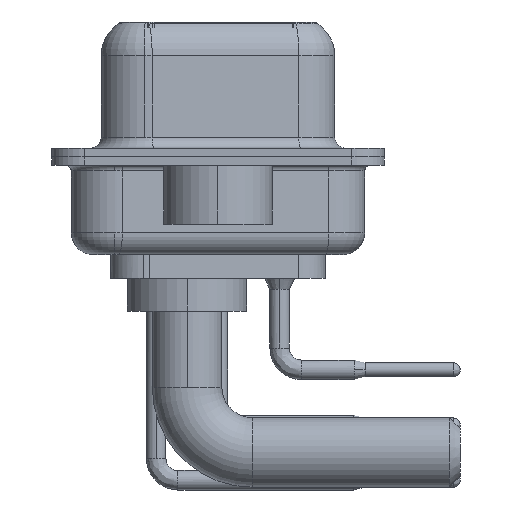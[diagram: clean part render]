
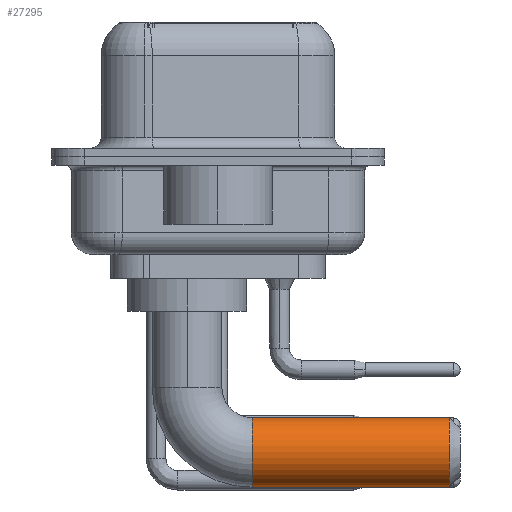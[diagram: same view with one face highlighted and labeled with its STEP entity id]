
A CAD part, left-side view. The second image highlights one B-rep face of the part: STEP entity #27295.
In plain terms, the highlighted cylindrical face has radius 1.6 mm (diameter 3.2 mm), a partial arc.
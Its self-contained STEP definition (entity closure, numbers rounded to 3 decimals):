
#317 = CARTESIAN_POINT ( 'NONE',  ( 0., -12.07, -8.1 ) ) ;
#1496 = DIRECTION ( 'NONE',  ( 0., -1., 0. ) ) ;
#2764 = ORIENTED_EDGE ( 'NONE', *, *, #27923, .F. ) ;
#2910 = DIRECTION ( 'NONE',  ( 0., 1., 0. ) ) ;
#3071 = DIRECTION ( 'NONE',  ( 0., -1., 0. ) ) ;
#3340 = VECTOR ( 'NONE', #7880, 1000. ) ;
#6502 = VERTEX_POINT ( 'NONE', #18603 ) ;
#7880 = DIRECTION ( 'NONE',  ( 0., -1., 0. ) ) ;
#8412 = CARTESIAN_POINT ( 'NONE',  ( 0., -3., -6.5 ) ) ;
#8477 = ORIENTED_EDGE ( 'NONE', *, *, #17776, .T. ) ;
#10902 = CYLINDRICAL_SURFACE ( 'NONE', #23457, 1.6 ) ;
#12902 = CIRCLE ( 'NONE', #27639, 1.6 ) ;
#13142 = LINE ( 'NONE', #25491, #16117 ) ;
#13550 = DIRECTION ( 'NONE',  ( 0., 0., -1. ) ) ;
#13879 = DIRECTION ( 'NONE',  ( -1., 0., 0. ) ) ;
#15323 = LINE ( 'NONE', #32443, #3340 ) ;
#15745 = EDGE_CURVE ( 'NONE', #6502, #26063, #15323, .T. ) ;
#16117 = VECTOR ( 'NONE', #3071, 1000. ) ;
#16149 = ORIENTED_EDGE ( 'NONE', *, *, #15745, .T. ) ;
#16342 = FACE_OUTER_BOUND ( 'NONE', #27611, .T. ) ;
#17776 = EDGE_CURVE ( 'NONE', #21153, #6502, #24983, .T. ) ;
#18603 = CARTESIAN_POINT ( 'NONE',  ( 0., -3., -8.1 ) ) ;
#18616 = EDGE_CURVE ( 'NONE', #26063, #27209, #12902, .T. ) ;
#20540 = CARTESIAN_POINT ( 'NONE',  ( 0., -12.07, -6.5 ) ) ;
#20944 = CARTESIAN_POINT ( 'NONE',  ( 0., -3., -6.5 ) ) ;
#21153 = VERTEX_POINT ( 'NONE', #28575 ) ;
#23457 = AXIS2_PLACEMENT_3D ( 'NONE', #20944, #30988, #13550 ) ;
#24983 = CIRCLE ( 'NONE', #29198, 1.6 ) ;
#25491 = CARTESIAN_POINT ( 'NONE',  ( 0., -3., -4.9 ) ) ;
#26063 = VERTEX_POINT ( 'NONE', #317 ) ;
#27209 = VERTEX_POINT ( 'NONE', #31150 ) ;
#27295 = ADVANCED_FACE ( 'NONE', ( #16342 ), #10902, .T. ) ;
#27611 = EDGE_LOOP ( 'NONE', ( #2764, #8477, #16149, #28631 ) ) ;
#27639 = AXIS2_PLACEMENT_3D ( 'NONE', #20540, #2910, #32412 ) ;
#27923 = EDGE_CURVE ( 'NONE', #21153, #27209, #13142, .T. ) ;
#28575 = CARTESIAN_POINT ( 'NONE',  ( 0., -3., -4.9 ) ) ;
#28631 = ORIENTED_EDGE ( 'NONE', *, *, #18616, .T. ) ;
#29198 = AXIS2_PLACEMENT_3D ( 'NONE', #8412, #1496, #13879 ) ;
#30988 = DIRECTION ( 'NONE',  ( 0., -1., 0. ) ) ;
#31150 = CARTESIAN_POINT ( 'NONE',  ( 0., -12.07, -4.9 ) ) ;
#32412 = DIRECTION ( 'NONE',  ( 0., 0., -1. ) ) ;
#32443 = CARTESIAN_POINT ( 'NONE',  ( 0., -3., -8.1 ) ) ;
